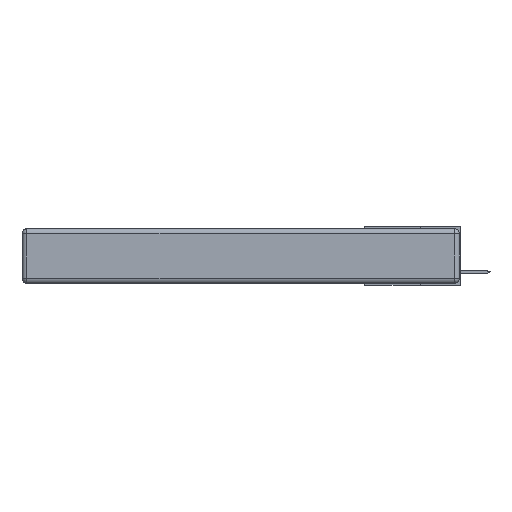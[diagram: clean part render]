
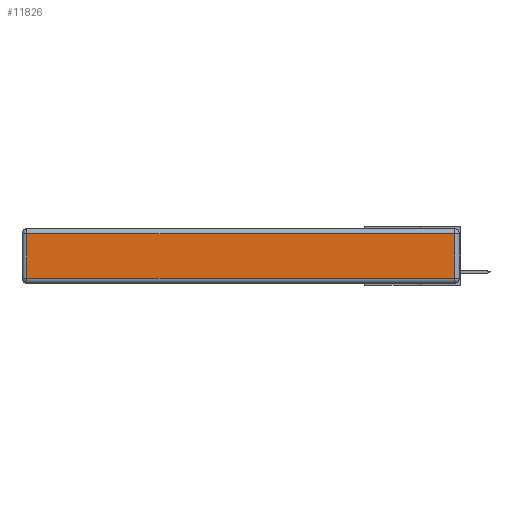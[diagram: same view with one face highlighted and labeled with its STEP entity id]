
A CAD part, left-side view. The second image highlights one B-rep face of the part: STEP entity #11826.
In plain terms, the highlighted planar face has unit normal (-1, 0, 0).
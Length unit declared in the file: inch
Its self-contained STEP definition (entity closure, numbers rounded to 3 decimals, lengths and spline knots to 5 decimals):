
#651 = VECTOR ( 'NONE', #5836, 39.37008 ) ;
#715 = LINE ( 'NONE', #10154, #18723 ) ;
#1126 = VERTEX_POINT ( 'NONE', #2338 ) ;
#1311 = CARTESIAN_POINT ( 'NONE',  ( 0., 2.72, -0.313 ) ) ;
#2013 = CARTESIAN_POINT ( 'NONE',  ( 0., 0.03, -0.343 ) ) ;
#2189 = DIRECTION ( 'NONE',  ( 0., -1., 0. ) ) ;
#2338 = CARTESIAN_POINT ( 'NONE',  ( 0., 0.03, -0.03 ) ) ;
#3885 = ORIENTED_EDGE ( 'NONE', *, *, #21661, .T. ) ;
#4584 = EDGE_LOOP ( 'NONE', ( #7663, #11399, #23693, #3885 ) ) ;
#5157 = FACE_OUTER_BOUND ( 'NONE', #4584, .T. ) ;
#5656 = CARTESIAN_POINT ( 'NONE',  ( 0., 2.72, -0.343 ) ) ;
#5726 = CARTESIAN_POINT ( 'NONE',  ( 0., 2.75, -0.03 ) ) ;
#5836 = DIRECTION ( 'NONE',  ( 0., 0., -1. ) ) ;
#5939 = DIRECTION ( 'NONE',  ( 0., 0., 1. ) ) ;
#6222 = EDGE_CURVE ( 'NONE', #1126, #10321, #12446, .T. ) ;
#7663 = ORIENTED_EDGE ( 'NONE', *, *, #16166, .T. ) ;
#10039 = CARTESIAN_POINT ( 'NONE',  ( 0., 0., -0.343 ) ) ;
#10154 = CARTESIAN_POINT ( 'NONE',  ( 0., 0., -0.313 ) ) ;
#10321 = VERTEX_POINT ( 'NONE', #25253 ) ;
#11399 = ORIENTED_EDGE ( 'NONE', *, *, #23068, .T. ) ;
#11826 = ADVANCED_FACE ( 'NONE', ( #5157 ), #22130, .T. ) ;
#12074 = DIRECTION ( 'NONE',  ( -1., 0., 0. ) ) ;
#12446 = LINE ( 'NONE', #5726, #16557 ) ;
#14114 = DIRECTION ( 'NONE',  ( 0., 0., 1. ) ) ;
#15924 = DIRECTION ( 'NONE',  ( 0., 1., 0. ) ) ;
#16166 = EDGE_CURVE ( 'NONE', #16500, #17774, #715, .T. ) ;
#16500 = VERTEX_POINT ( 'NONE', #1311 ) ;
#16557 = VECTOR ( 'NONE', #15924, 39.37008 ) ;
#17699 = LINE ( 'NONE', #5656, #651 ) ;
#17774 = VERTEX_POINT ( 'NONE', #21812 ) ;
#18723 = VECTOR ( 'NONE', #2189, 39.37008 ) ;
#21661 = EDGE_CURVE ( 'NONE', #10321, #16500, #17699, .T. ) ;
#21812 = CARTESIAN_POINT ( 'NONE',  ( 0., 0.03, -0.313 ) ) ;
#22031 = LINE ( 'NONE', #2013, #22344 ) ;
#22130 = PLANE ( 'NONE',  #24332 ) ;
#22344 = VECTOR ( 'NONE', #5939, 39.37008 ) ;
#23068 = EDGE_CURVE ( 'NONE', #17774, #1126, #22031, .T. ) ;
#23693 = ORIENTED_EDGE ( 'NONE', *, *, #6222, .T. ) ;
#24332 = AXIS2_PLACEMENT_3D ( 'NONE', #10039, #12074, #14114 ) ;
#25253 = CARTESIAN_POINT ( 'NONE',  ( 0., 2.72, -0.03 ) ) ;
